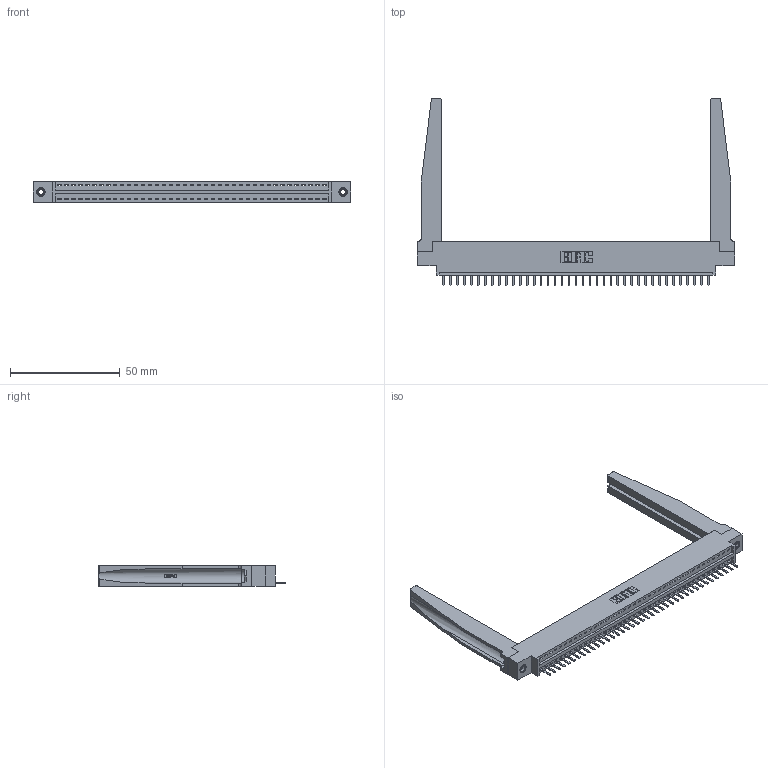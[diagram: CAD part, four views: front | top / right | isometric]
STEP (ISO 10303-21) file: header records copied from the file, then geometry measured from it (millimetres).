
FILE_DESCRIPTION (( 'STEP AP203' ), '1' );
FILE_NAME ('396-039-520-678.STEP', '2019-10-27T18:57:54', ( '' ), ( '' ), 'SwSTEP 2.0', 'SolidWorks 2016', '' );
FILE_SCHEMA (( 'CONFIG_CONTROL_DESIGN' ));
Length unit declared in the file: inch
Products named in the file (5): 346-220-078_345-220-078; 345-292-001_345-293-120; 396-039-520-678; 345-250-001_345-250-001-102; 346 Part_0.170 Offset - 0.156 Dia-TH
Assembly tree (44 placements, depth 2):
  396-039-520-678
    346 Part_0.170 Offset - 0.156 Dia-TH
    345-292-001_345-293-120  x39
    346-220-078_345-220-078  x2
    345-250-001_345-250-001-102  x2
Bounding box: 144.4 x 85.29 x 9.4 mm (x, y, z)
Volume: 20443.6 mm3; surface area: 23210.2 mm2
Topology: 44 solids, 44 shells, 2778 faces, 8125 edges, 5302 vertices
Faces by surface type: plane 1860, cylinder 866, bspline 36, cone 12, torus 4
Entity records: 29602 total; most frequent: CARTESIAN_POINT 6000, ORIENTED_EDGE 4850, DIRECTION 4269, EDGE_CURVE 2425, VECTOR 2039, LINE 2039, VERTEX_POINT 1608, AXIS2_PLACEMENT_3D 1115
